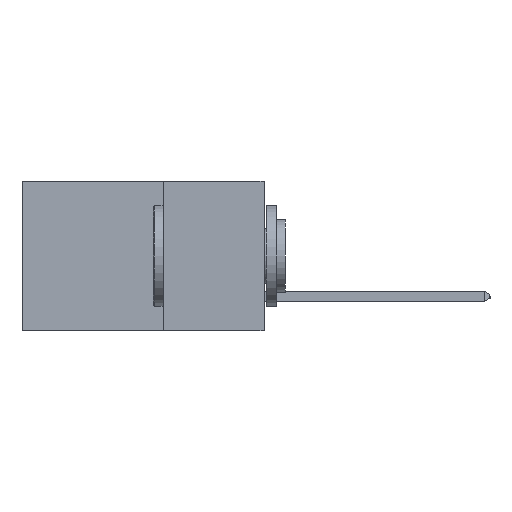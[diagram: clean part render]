
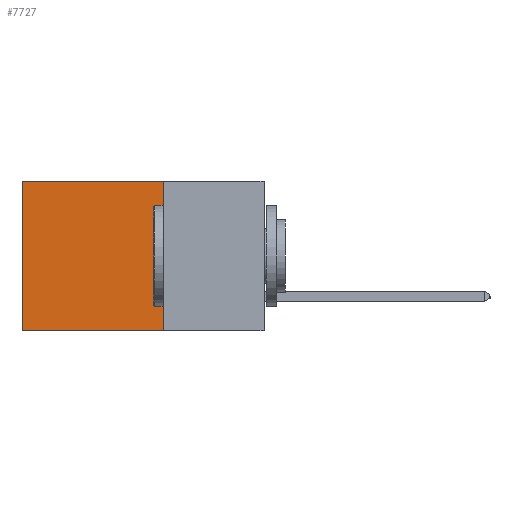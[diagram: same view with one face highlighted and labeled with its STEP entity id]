
A CAD part, left-side view. The second image highlights one B-rep face of the part: STEP entity #7727.
In plain terms, the highlighted planar face has unit normal (-1, 0, 0).
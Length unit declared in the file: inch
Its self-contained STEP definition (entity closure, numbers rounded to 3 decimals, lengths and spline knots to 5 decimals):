
#486 = DIRECTION ( 'NONE',  ( 0., 1., 0. ) ) ;
#791 = ORIENTED_EDGE ( 'NONE', *, *, #4334, .F. ) ;
#838 = DIRECTION ( 'NONE',  ( 0., 1., 0. ) ) ;
#1382 = VERTEX_POINT ( 'NONE', #1443 ) ;
#1443 = CARTESIAN_POINT ( 'NONE',  ( 0.298, 0.25, 0. ) ) ;
#2207 = PLANE ( 'NONE',  #9409 ) ;
#2354 = LINE ( 'NONE', #14253, #5450 ) ;
#2652 = LINE ( 'NONE', #8865, #5385 ) ;
#2834 = ORIENTED_EDGE ( 'NONE', *, *, #10388, .F. ) ;
#3601 = LINE ( 'NONE', #4711, #8968 ) ;
#4334 = EDGE_CURVE ( 'NONE', #6602, #13792, #8368, .T. ) ;
#4536 = DIRECTION ( 'NONE',  ( 1., 0., 0. ) ) ;
#4711 = CARTESIAN_POINT ( 'NONE',  ( 0.298, 0.25, 0. ) ) ;
#5385 = VECTOR ( 'NONE', #838, 39.37008 ) ;
#5450 = VECTOR ( 'NONE', #6412, 39.37008 ) ;
#5455 = EDGE_LOOP ( 'NONE', ( #6013, #791, #2834, #9141 ) ) ;
#5640 = CARTESIAN_POINT ( 'NONE',  ( 0.298, 0.25, -0.37 ) ) ;
#5889 = DIRECTION ( 'NONE',  ( 0., 0., -1. ) ) ;
#6013 = ORIENTED_EDGE ( 'NONE', *, *, #8142, .T. ) ;
#6412 = DIRECTION ( 'NONE',  ( 0., 0., -1. ) ) ;
#6602 = VERTEX_POINT ( 'NONE', #10598 ) ;
#7727 = ADVANCED_FACE ( 'NONE', ( #11107 ), #2207, .F. ) ;
#8014 = VECTOR ( 'NONE', #486, 39.37008 ) ;
#8142 = EDGE_CURVE ( 'NONE', #11830, #13792, #2354, .T. ) ;
#8368 = LINE ( 'NONE', #5640, #8014 ) ;
#8865 = CARTESIAN_POINT ( 'NONE',  ( 0.298, 0.25, 0. ) ) ;
#8968 = VECTOR ( 'NONE', #5889, 39.37008 ) ;
#9141 = ORIENTED_EDGE ( 'NONE', *, *, #10165, .T. ) ;
#9409 = AXIS2_PLACEMENT_3D ( 'NONE', #11283, #4536, #12479 ) ;
#9641 = CARTESIAN_POINT ( 'NONE',  ( 0.298, 0.6, -0.37 ) ) ;
#10165 = EDGE_CURVE ( 'NONE', #1382, #11830, #2652, .T. ) ;
#10388 = EDGE_CURVE ( 'NONE', #1382, #6602, #3601, .T. ) ;
#10598 = CARTESIAN_POINT ( 'NONE',  ( 0.298, 0.25, -0.37 ) ) ;
#11107 = FACE_OUTER_BOUND ( 'NONE', #5455, .T. ) ;
#11283 = CARTESIAN_POINT ( 'NONE',  ( 0.298, 0.25, 0. ) ) ;
#11830 = VERTEX_POINT ( 'NONE', #14394 ) ;
#12479 = DIRECTION ( 'NONE',  ( 0., 0., -1. ) ) ;
#13792 = VERTEX_POINT ( 'NONE', #9641 ) ;
#14253 = CARTESIAN_POINT ( 'NONE',  ( 0.298, 0.6, 0. ) ) ;
#14394 = CARTESIAN_POINT ( 'NONE',  ( 0.298, 0.6, 0. ) ) ;
